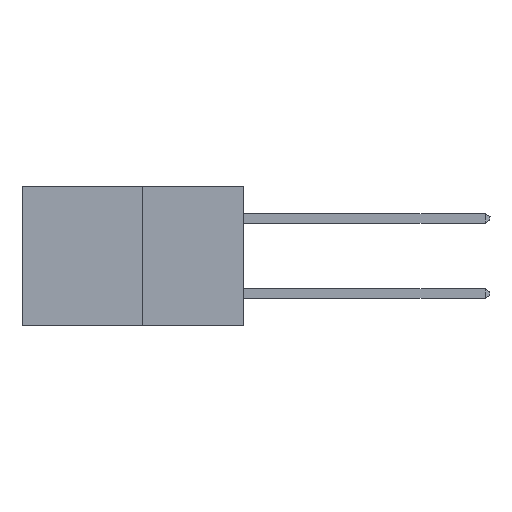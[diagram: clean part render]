
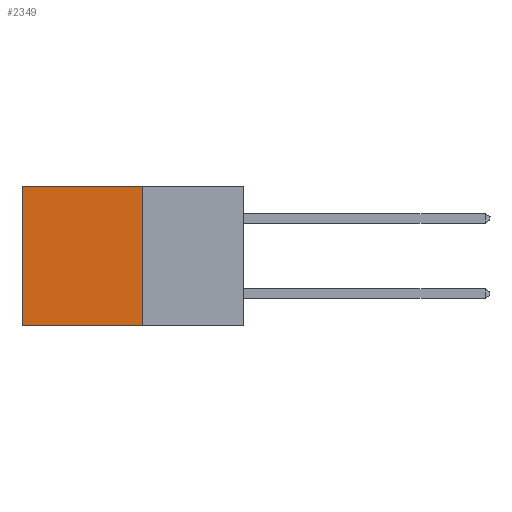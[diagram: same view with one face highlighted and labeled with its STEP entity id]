
A CAD part, left-side view. The second image highlights one B-rep face of the part: STEP entity #2349.
In plain terms, the highlighted planar face has unit normal (-1, 0, 0).
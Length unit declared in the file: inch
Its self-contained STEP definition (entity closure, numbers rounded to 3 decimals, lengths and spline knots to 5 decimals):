
#604 = VECTOR ( 'NONE', #5790, 39.37008 ) ;
#1178 = CARTESIAN_POINT ( 'NONE',  ( 0.277, 0.59, 0. ) ) ;
#1248 = CARTESIAN_POINT ( 'NONE',  ( 0.277, 0.59, -0.37 ) ) ;
#1289 = AXIS2_PLACEMENT_3D ( 'NONE', #6248, #2648, #5116 ) ;
#1830 = VERTEX_POINT ( 'NONE', #4950 ) ;
#1895 = DIRECTION ( 'NONE',  ( 0., 1., 0. ) ) ;
#2125 = ORIENTED_EDGE ( 'NONE', *, *, #8131, .T. ) ;
#2349 = ADVANCED_FACE ( 'NONE', ( #8881 ), #3913, .F. ) ;
#2604 = EDGE_CURVE ( 'NONE', #4885, #3759, #4764, .T. ) ;
#2648 = DIRECTION ( 'NONE',  ( 1., 0., 0. ) ) ;
#2745 = ORIENTED_EDGE ( 'NONE', *, *, #7897, .F. ) ;
#2983 = LINE ( 'NONE', #1248, #4625 ) ;
#3399 = CARTESIAN_POINT ( 'NONE',  ( 0.277, 0.59, -0.37 ) ) ;
#3759 = VERTEX_POINT ( 'NONE', #3399 ) ;
#3881 = ORIENTED_EDGE ( 'NONE', *, *, #2604, .F. ) ;
#3913 = PLANE ( 'NONE',  #1289 ) ;
#4185 = ORIENTED_EDGE ( 'NONE', *, *, #5670, .T. ) ;
#4290 = VERTEX_POINT ( 'NONE', #1178 ) ;
#4625 = VECTOR ( 'NONE', #8167, 39.37008 ) ;
#4648 = CARTESIAN_POINT ( 'NONE',  ( 0.277, 0.27, -0.37 ) ) ;
#4764 = LINE ( 'NONE', #6616, #4979 ) ;
#4885 = VERTEX_POINT ( 'NONE', #4648 ) ;
#4950 = CARTESIAN_POINT ( 'NONE',  ( 0.277, 0.27, 0. ) ) ;
#4979 = VECTOR ( 'NONE', #6455, 39.37008 ) ;
#5116 = DIRECTION ( 'NONE',  ( 0., 0., -1. ) ) ;
#5670 = EDGE_CURVE ( 'NONE', #4290, #3759, #2983, .T. ) ;
#5677 = VECTOR ( 'NONE', #1895, 39.37008 ) ;
#5790 = DIRECTION ( 'NONE',  ( 0., 0., -1. ) ) ;
#5884 = LINE ( 'NONE', #7448, #5677 ) ;
#6248 = CARTESIAN_POINT ( 'NONE',  ( 0.277, 0.27, -0.37 ) ) ;
#6455 = DIRECTION ( 'NONE',  ( 0., 1., 0. ) ) ;
#6616 = CARTESIAN_POINT ( 'NONE',  ( 0.277, 0.27, -0.37 ) ) ;
#7448 = CARTESIAN_POINT ( 'NONE',  ( 0.277, 0.27, 0. ) ) ;
#7721 = EDGE_LOOP ( 'NONE', ( #4185, #3881, #2745, #2125 ) ) ;
#7786 = LINE ( 'NONE', #7814, #604 ) ;
#7814 = CARTESIAN_POINT ( 'NONE',  ( 0.277, 0.27, -0.37 ) ) ;
#7897 = EDGE_CURVE ( 'NONE', #1830, #4885, #7786, .T. ) ;
#8131 = EDGE_CURVE ( 'NONE', #1830, #4290, #5884, .T. ) ;
#8167 = DIRECTION ( 'NONE',  ( 0., 0., -1. ) ) ;
#8881 = FACE_OUTER_BOUND ( 'NONE', #7721, .T. ) ;
